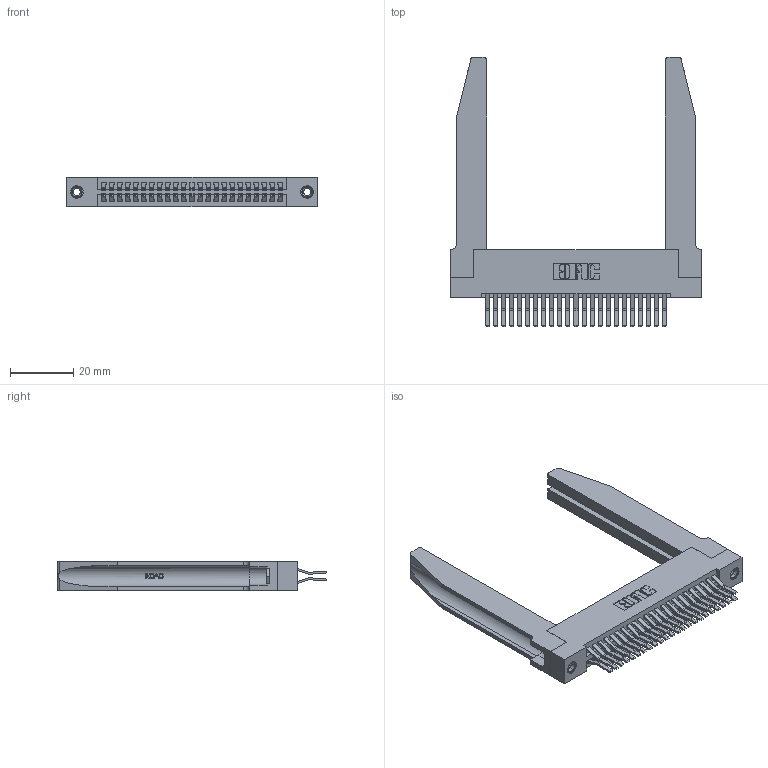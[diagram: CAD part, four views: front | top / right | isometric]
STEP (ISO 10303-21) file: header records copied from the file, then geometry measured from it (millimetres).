
FILE_DESCRIPTION (( 'STEP AP203' ), '1' );
FILE_NAME ('345-046-560-278.STEP', '2019-10-29T03:25:25', ( '' ), ( '' ), 'SwSTEP 2.0', 'SolidWorks 2016', '' );
FILE_SCHEMA (( 'CONFIG_CONTROL_DESIGN' ));
Length unit declared in the file: inch
Products named in the file (5): 345-220-078_345-220-078; 345 Part_Flush Mounting Lugs - 0.156 Dia-TH; 345-292-001_560 Tail; 345-250-001_345-250-001-102; 345-046-560-278
Assembly tree (51 placements, depth 2):
  345-046-560-278
    345 Part_Flush Mounting Lugs - 0.156 Dia-TH
    345-292-001_560 Tail  x46
    345-250-001_345-250-001-102  x2
    345-220-078_345-220-078  x2
Bounding box: 79.65 x 85.41 x 9.4 mm (x, y, z)
Volume: 15633.3 mm3; surface area: 18868.5 mm2
Topology: 51 solids, 51 shells, 2752 faces, 8079 edges, 5314 vertices
Faces by surface type: plane 1740, cylinder 960, bspline 36, cone 12, torus 4
Entity records: 25432 total; most frequent: CARTESIAN_POINT 5199, ORIENTED_EDGE 4030, DIRECTION 3605, EDGE_CURVE 2015, VECTOR 1693, LINE 1693, VERTEX_POINT 1336, AXIS2_PLACEMENT_3D 956
